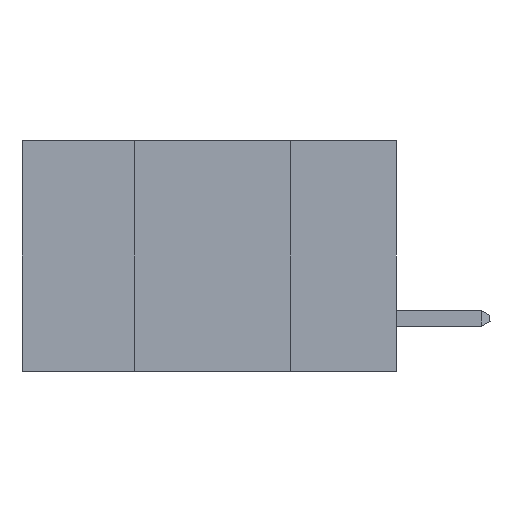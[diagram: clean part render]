
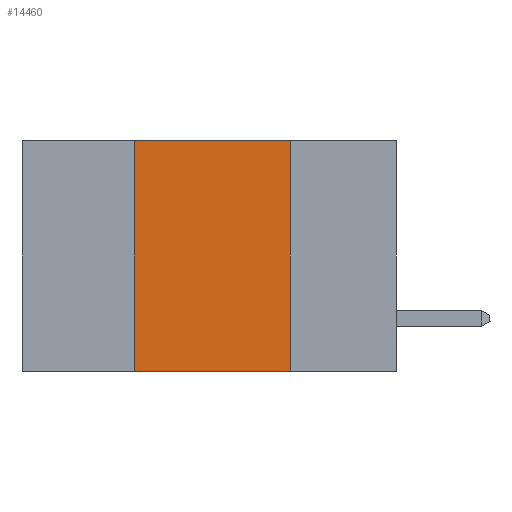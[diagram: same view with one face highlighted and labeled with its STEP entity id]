
A CAD part, left-side view. The second image highlights one B-rep face of the part: STEP entity #14460.
In plain terms, the highlighted planar face has unit normal (-1, 0, 0).
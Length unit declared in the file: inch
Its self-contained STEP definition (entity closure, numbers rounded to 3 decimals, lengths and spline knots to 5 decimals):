
#725 = CARTESIAN_POINT ( 'NONE',  ( 0., 0.42, 0. ) ) ;
#780 = PLANE ( 'NONE',  #3437 ) ;
#904 = DIRECTION ( 'NONE',  ( 0., -1., 0. ) ) ;
#1929 = CARTESIAN_POINT ( 'NONE',  ( 0., 0.17, -0.37 ) ) ;
#3437 = AXIS2_PLACEMENT_3D ( 'NONE', #10203, #11510, #3553 ) ;
#3553 = DIRECTION ( 'NONE',  ( 0., 0., -1. ) ) ;
#4349 = DIRECTION ( 'NONE',  ( 0., 0., 1. ) ) ;
#4886 = EDGE_CURVE ( 'NONE', #12736, #8037, #15475, .T. ) ;
#5096 = ORIENTED_EDGE ( 'NONE', *, *, #13731, .F. ) ;
#5449 = EDGE_CURVE ( 'NONE', #13746, #8037, #16639, .T. ) ;
#6262 = VECTOR ( 'NONE', #4349, 39.37008 ) ;
#6491 = CARTESIAN_POINT ( 'NONE',  ( 0., 0.42, -0.37 ) ) ;
#7692 = VECTOR ( 'NONE', #904, 39.37008 ) ;
#7868 = LINE ( 'NONE', #14182, #13998 ) ;
#8037 = VERTEX_POINT ( 'NONE', #1929 ) ;
#8498 = CARTESIAN_POINT ( 'NONE',  ( 0., 0.17, 0. ) ) ;
#8559 = ORIENTED_EDGE ( 'NONE', *, *, #5449, .F. ) ;
#9064 = CARTESIAN_POINT ( 'NONE',  ( 0., 0.6, -0.37 ) ) ;
#10203 = CARTESIAN_POINT ( 'NONE',  ( 0., 0.6, 0. ) ) ;
#10324 = DIRECTION ( 'NONE',  ( 0., -1., 0. ) ) ;
#11074 = CARTESIAN_POINT ( 'NONE',  ( 0., 0.42, 0. ) ) ;
#11510 = DIRECTION ( 'NONE',  ( 1., 0., 0. ) ) ;
#12204 = FACE_OUTER_BOUND ( 'NONE', #15858, .T. ) ;
#12736 = VERTEX_POINT ( 'NONE', #6491 ) ;
#13248 = LINE ( 'NONE', #11074, #6262 ) ;
#13622 = ORIENTED_EDGE ( 'NONE', *, *, #16475, .F. ) ;
#13731 = EDGE_CURVE ( 'NONE', #12736, #14422, #13248, .T. ) ;
#13746 = VERTEX_POINT ( 'NONE', #8498 ) ;
#13998 = VECTOR ( 'NONE', #10324, 39.37008 ) ;
#14182 = CARTESIAN_POINT ( 'NONE',  ( 0., 0.6, 0. ) ) ;
#14399 = DIRECTION ( 'NONE',  ( 0., 0., -1. ) ) ;
#14422 = VERTEX_POINT ( 'NONE', #725 ) ;
#14460 = ADVANCED_FACE ( 'NONE', ( #12204 ), #780, .F. ) ;
#14602 = CARTESIAN_POINT ( 'NONE',  ( 0., 0.17, 0. ) ) ;
#15475 = LINE ( 'NONE', #9064, #7692 ) ;
#15858 = EDGE_LOOP ( 'NONE', ( #8559, #13622, #5096, #16634 ) ) ;
#16234 = VECTOR ( 'NONE', #14399, 39.37008 ) ;
#16475 = EDGE_CURVE ( 'NONE', #14422, #13746, #7868, .T. ) ;
#16634 = ORIENTED_EDGE ( 'NONE', *, *, #4886, .T. ) ;
#16639 = LINE ( 'NONE', #14602, #16234 ) ;
